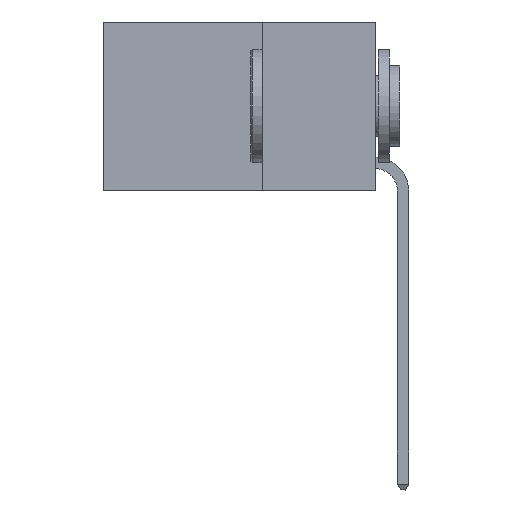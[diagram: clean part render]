
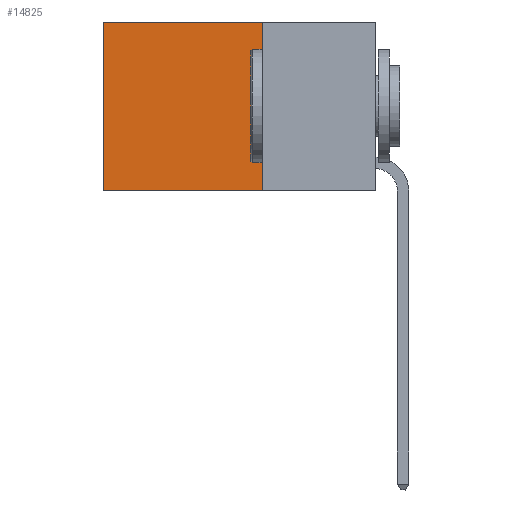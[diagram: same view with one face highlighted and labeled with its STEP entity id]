
A CAD part, left-side view. The second image highlights one B-rep face of the part: STEP entity #14825.
In plain terms, the highlighted planar face has unit normal (-1, 0, 0).
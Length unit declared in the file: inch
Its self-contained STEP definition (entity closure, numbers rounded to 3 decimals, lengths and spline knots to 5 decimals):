
#31 = EDGE_CURVE ( 'NONE', #4664, #19831, #11888, .T. ) ;
#257 = CARTESIAN_POINT ( 'NONE',  ( 0.2625, 0.25, 0. ) ) ;
#363 = DIRECTION ( 'NONE',  ( 0., 1., 0. ) ) ;
#1032 = DIRECTION ( 'NONE',  ( 0., 0., -1. ) ) ;
#1248 = VECTOR ( 'NONE', #16378, 39.37008 ) ;
#2351 = VECTOR ( 'NONE', #363, 39.37008 ) ;
#2584 = EDGE_CURVE ( 'NONE', #12248, #3362, #17846, .T. ) ;
#3362 = VERTEX_POINT ( 'NONE', #4907 ) ;
#3517 = ORIENTED_EDGE ( 'NONE', *, *, #31, .F. ) ;
#4664 = VERTEX_POINT ( 'NONE', #5779 ) ;
#4907 = CARTESIAN_POINT ( 'NONE',  ( 0.2625, 0.6, -0.37 ) ) ;
#4920 = AXIS2_PLACEMENT_3D ( 'NONE', #8654, #12357, #1032 ) ;
#5056 = VECTOR ( 'NONE', #6716, 39.37008 ) ;
#5779 = CARTESIAN_POINT ( 'NONE',  ( 0.2625, 0.25, 0. ) ) ;
#6416 = EDGE_CURVE ( 'NONE', #4664, #12248, #8302, .T. ) ;
#6716 = DIRECTION ( 'NONE',  ( 0., 0., -1. ) ) ;
#6738 = EDGE_LOOP ( 'NONE', ( #19980, #16067, #3517, #10773 ) ) ;
#6822 = LINE ( 'NONE', #8505, #15902 ) ;
#6957 = CARTESIAN_POINT ( 'NONE',  ( 0.2625, 0.6, 0. ) ) ;
#8302 = LINE ( 'NONE', #257, #2351 ) ;
#8306 = CARTESIAN_POINT ( 'NONE',  ( 0.2625, 0.25, 0. ) ) ;
#8505 = CARTESIAN_POINT ( 'NONE',  ( 0.2625, 0.25, -0.37 ) ) ;
#8654 = CARTESIAN_POINT ( 'NONE',  ( 0.2625, 0.25, 0. ) ) ;
#8865 = PLANE ( 'NONE',  #4920 ) ;
#10773 = ORIENTED_EDGE ( 'NONE', *, *, #6416, .T. ) ;
#11888 = LINE ( 'NONE', #8306, #5056 ) ;
#12248 = VERTEX_POINT ( 'NONE', #18463 ) ;
#12357 = DIRECTION ( 'NONE',  ( 1., 0., 0. ) ) ;
#13266 = DIRECTION ( 'NONE',  ( 0., 1., 0. ) ) ;
#14825 = ADVANCED_FACE ( 'NONE', ( #19875 ), #8865, .F. ) ;
#15902 = VECTOR ( 'NONE', #13266, 39.37008 ) ;
#16067 = ORIENTED_EDGE ( 'NONE', *, *, #20274, .F. ) ;
#16378 = DIRECTION ( 'NONE',  ( 0., 0., -1. ) ) ;
#17836 = CARTESIAN_POINT ( 'NONE',  ( 0.2625, 0.25, -0.37 ) ) ;
#17846 = LINE ( 'NONE', #6957, #1248 ) ;
#18463 = CARTESIAN_POINT ( 'NONE',  ( 0.2625, 0.6, 0. ) ) ;
#19831 = VERTEX_POINT ( 'NONE', #17836 ) ;
#19875 = FACE_OUTER_BOUND ( 'NONE', #6738, .T. ) ;
#19980 = ORIENTED_EDGE ( 'NONE', *, *, #2584, .T. ) ;
#20274 = EDGE_CURVE ( 'NONE', #19831, #3362, #6822, .T. ) ;
